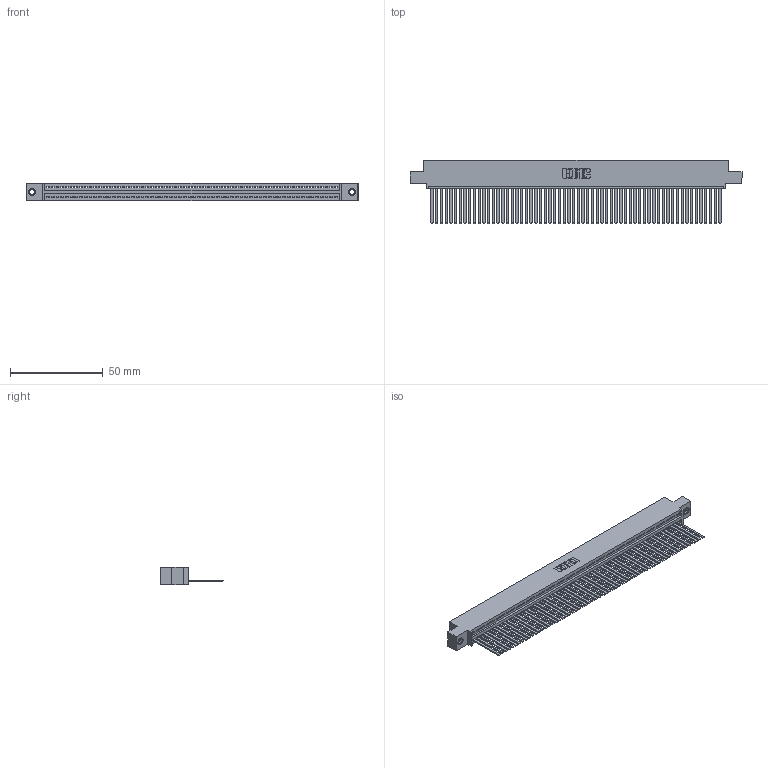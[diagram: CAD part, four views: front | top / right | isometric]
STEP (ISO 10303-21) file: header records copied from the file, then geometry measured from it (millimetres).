
FILE_DESCRIPTION (( 'STEP AP203' ), '1' );
FILE_NAME ('395-062-544-407.STEP', '2018-11-24T04:24:08', ( '' ), ( '' ), 'SwSTEP 2.0', 'SolidWorks 2016', '' );
FILE_SCHEMA (( 'CONFIG_CONTROL_DESIGN' ));
Length unit declared in the file: inch
Products named in the file (4): 345-292-001_345-293-144; 345-250-001_345-250-005-103; 395-062-544-407; 345 Part_0.110 Offset - 0.156 Dia-TI
Assembly tree (65 placements, depth 2):
  395-062-544-407
    345 Part_0.110 Offset - 0.156 Dia-TI
    345-292-001_345-293-144  x62
    345-250-001_345-250-005-103  x2
Bounding box: 178.69 x 33.96 x 9.4 mm (x, y, z)
Volume: 17767.1 mm3; surface area: 26152.7 mm2
Topology: 65 solids, 65 shells, 3414 faces, 10285 edges, 6766 vertices
Faces by surface type: plane 2348, cylinder 1050, cone 12, torus 4
Entity records: 45104 total; most frequent: CARTESIAN_POINT 7793, ORIENTED_EDGE 7782, DIRECTION 6801, EDGE_CURVE 3891, VECTOR 3495, LINE 3495, VERTEX_POINT 2588, AXIS2_PLACEMENT_3D 1653
